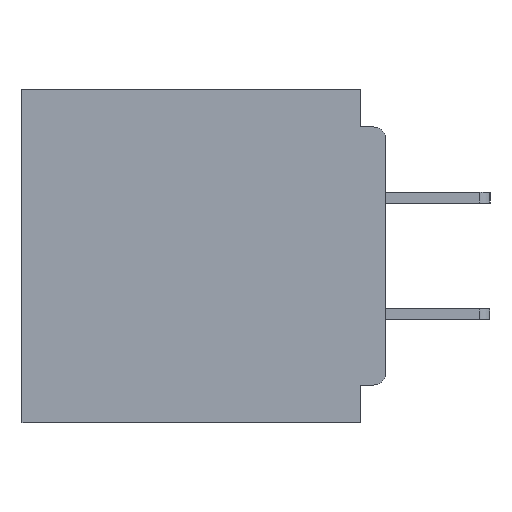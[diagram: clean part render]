
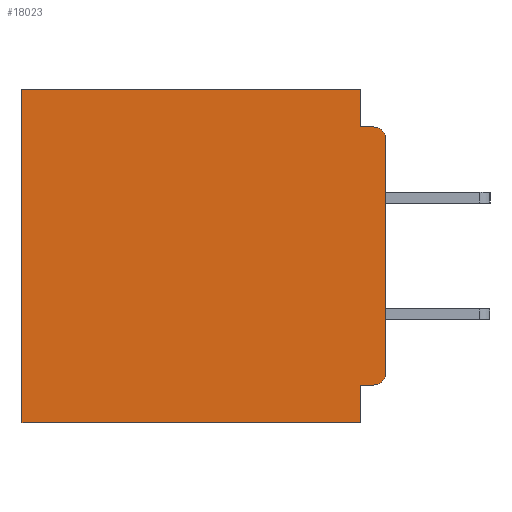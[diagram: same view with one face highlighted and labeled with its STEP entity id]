
A CAD part, left-side view. The second image highlights one B-rep face of the part: STEP entity #18023.
In plain terms, the highlighted planar face has unit normal (-1, 0, 0).
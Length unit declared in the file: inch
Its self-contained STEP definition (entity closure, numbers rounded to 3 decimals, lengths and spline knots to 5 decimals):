
#445 = EDGE_CURVE ( 'NONE', #33540, #35235, #53039, .T. ) ;
#1451 = CARTESIAN_POINT ( 'NONE',  ( 0.3, 0., -0.4 ) ) ;
#1648 = CARTESIAN_POINT ( 'NONE',  ( 0.3, 0., -0.4 ) ) ;
#2096 = ORIENTED_EDGE ( 'NONE', *, *, #445, .T. ) ;
#2358 = VECTOR ( 'NONE', #5989, 39.37008 ) ;
#2454 = VERTEX_POINT ( 'NONE', #12246 ) ;
#2804 = DIRECTION ( 'NONE',  ( 0., 0., -1. ) ) ;
#3564 = VERTEX_POINT ( 'NONE', #42835 ) ;
#4444 = DIRECTION ( 'NONE',  ( 0., 0., -1. ) ) ;
#5165 = EDGE_CURVE ( 'NONE', #33540, #9304, #45964, .T. ) ;
#5500 = LINE ( 'NONE', #1451, #48750 ) ;
#5989 = DIRECTION ( 'NONE',  ( 0., 1., 0. ) ) ;
#7007 = CARTESIAN_POINT ( 'NONE',  ( 0.3, 0.015, -0.045 ) ) ;
#7135 = VECTOR ( 'NONE', #4444, 39.37008 ) ;
#8494 = LINE ( 'NONE', #13197, #7135 ) ;
#8548 = LINE ( 'NONE', #48949, #30179 ) ;
#9304 = VERTEX_POINT ( 'NONE', #12544 ) ;
#10803 = EDGE_CURVE ( 'NONE', #35089, #15074, #8494, .T. ) ;
#12246 = CARTESIAN_POINT ( 'NONE',  ( 0.3, 0.437, 0. ) ) ;
#12320 = AXIS2_PLACEMENT_3D ( 'NONE', #33677, #44845, #49790 ) ;
#12544 = CARTESIAN_POINT ( 'NONE',  ( 0.3, 0.031, -0.355 ) ) ;
#13197 = CARTESIAN_POINT ( 'NONE',  ( 0.3, 0.031, 0. ) ) ;
#13611 = DIRECTION ( 'NONE',  ( -1., 0., 0. ) ) ;
#14732 = EDGE_CURVE ( 'NONE', #35089, #2454, #47645, .T. ) ;
#15074 = VERTEX_POINT ( 'NONE', #53168 ) ;
#16512 = EDGE_CURVE ( 'NONE', #40631, #35235, #5500, .T. ) ;
#17416 = DIRECTION ( 'NONE',  ( 0., 1., 0. ) ) ;
#17921 = VECTOR ( 'NONE', #17416, 39.37008 ) ;
#18023 = ADVANCED_FACE ( 'NONE', ( #47334 ), #24431, .F. ) ;
#19480 = ORIENTED_EDGE ( 'NONE', *, *, #38694, .F. ) ;
#20081 = ORIENTED_EDGE ( 'NONE', *, *, #14732, .T. ) ;
#20092 = CARTESIAN_POINT ( 'NONE',  ( 0.3, 0., -0.4 ) ) ;
#20930 = CARTESIAN_POINT ( 'NONE',  ( 0.3, 0., -0.06 ) ) ;
#21140 = ORIENTED_EDGE ( 'NONE', *, *, #53296, .F. ) ;
#23160 = DIRECTION ( 'NONE',  ( 0., 0., -1. ) ) ;
#24431 = PLANE ( 'NONE',  #30655 ) ;
#24699 = CARTESIAN_POINT ( 'NONE',  ( 0.3, 0.437, -0.4 ) ) ;
#24722 = VECTOR ( 'NONE', #46627, 39.37008 ) ;
#25220 = EDGE_LOOP ( 'NONE', ( #27662, #39268, #21140, #50138, #20081, #36239, #19480, #35640, #35937, #2096 ) ) ;
#25744 = VECTOR ( 'NONE', #46243, 39.37008 ) ;
#26354 = AXIS2_PLACEMENT_3D ( 'NONE', #39465, #13611, #43816 ) ;
#26594 = EDGE_CURVE ( 'NONE', #40631, #32917, #36725, .T. ) ;
#27662 = ORIENTED_EDGE ( 'NONE', *, *, #16512, .F. ) ;
#28474 = CARTESIAN_POINT ( 'NONE',  ( 0.3, 0.015, -0.355 ) ) ;
#28716 = DIRECTION ( 'NONE',  ( 1., 0., 0. ) ) ;
#30179 = VECTOR ( 'NONE', #23160, 39.37008 ) ;
#30190 = CARTESIAN_POINT ( 'NONE',  ( 0.3, 0., -0.355 ) ) ;
#30655 = AXIS2_PLACEMENT_3D ( 'NONE', #20092, #28716, #2804 ) ;
#32323 = EDGE_CURVE ( 'NONE', #2454, #3564, #42192, .T. ) ;
#32917 = VERTEX_POINT ( 'NONE', #7007 ) ;
#33337 = DIRECTION ( 'NONE',  ( 0., 0., -1. ) ) ;
#33540 = VERTEX_POINT ( 'NONE', #28474 ) ;
#33677 = CARTESIAN_POINT ( 'NONE',  ( 0.3, 0.015, -0.34 ) ) ;
#35089 = VERTEX_POINT ( 'NONE', #39679 ) ;
#35235 = VERTEX_POINT ( 'NONE', #44947 ) ;
#35640 = ORIENTED_EDGE ( 'NONE', *, *, #55231, .F. ) ;
#35937 = ORIENTED_EDGE ( 'NONE', *, *, #5165, .F. ) ;
#36239 = ORIENTED_EDGE ( 'NONE', *, *, #32323, .T. ) ;
#36725 = CIRCLE ( 'NONE', #26354, 0.015 ) ;
#36885 = LINE ( 'NONE', #1648, #2358 ) ;
#38694 = EDGE_CURVE ( 'NONE', #44378, #3564, #36885, .T. ) ;
#39268 = ORIENTED_EDGE ( 'NONE', *, *, #26594, .T. ) ;
#39465 = CARTESIAN_POINT ( 'NONE',  ( 0.3, 0.015, -0.06 ) ) ;
#39679 = CARTESIAN_POINT ( 'NONE',  ( 0.3, 0.031, 0. ) ) ;
#40631 = VERTEX_POINT ( 'NONE', #20930 ) ;
#41902 = CARTESIAN_POINT ( 'NONE',  ( 0.3, 0., -0.045 ) ) ;
#42192 = LINE ( 'NONE', #24699, #52275 ) ;
#42306 = CARTESIAN_POINT ( 'NONE',  ( 0.3, 0., 0. ) ) ;
#42835 = CARTESIAN_POINT ( 'NONE',  ( 0.3, 0.437, -0.4 ) ) ;
#43816 = DIRECTION ( 'NONE',  ( 0., 0., -1. ) ) ;
#44378 = VERTEX_POINT ( 'NONE', #54559 ) ;
#44555 = DIRECTION ( 'NONE',  ( 0., 0., -1. ) ) ;
#44845 = DIRECTION ( 'NONE',  ( -1., 0., 0. ) ) ;
#44947 = CARTESIAN_POINT ( 'NONE',  ( 0.3, 0., -0.34 ) ) ;
#45964 = LINE ( 'NONE', #30190, #17921 ) ;
#46243 = DIRECTION ( 'NONE',  ( 0., -1., 0. ) ) ;
#46627 = DIRECTION ( 'NONE',  ( 0., 1., 0. ) ) ;
#47334 = FACE_OUTER_BOUND ( 'NONE', #25220, .T. ) ;
#47645 = LINE ( 'NONE', #42306, #24722 ) ;
#48637 = LINE ( 'NONE', #41902, #25744 ) ;
#48750 = VECTOR ( 'NONE', #44555, 39.37008 ) ;
#48949 = CARTESIAN_POINT ( 'NONE',  ( 0.3, 0.031, -0.4 ) ) ;
#49790 = DIRECTION ( 'NONE',  ( 0., 0., -1. ) ) ;
#50138 = ORIENTED_EDGE ( 'NONE', *, *, #10803, .F. ) ;
#52275 = VECTOR ( 'NONE', #33337, 39.37008 ) ;
#53039 = CIRCLE ( 'NONE', #12320, 0.015 ) ;
#53168 = CARTESIAN_POINT ( 'NONE',  ( 0.3, 0.031, -0.045 ) ) ;
#53296 = EDGE_CURVE ( 'NONE', #15074, #32917, #48637, .T. ) ;
#54559 = CARTESIAN_POINT ( 'NONE',  ( 0.3, 0.031, -0.4 ) ) ;
#55231 = EDGE_CURVE ( 'NONE', #9304, #44378, #8548, .T. ) ;
